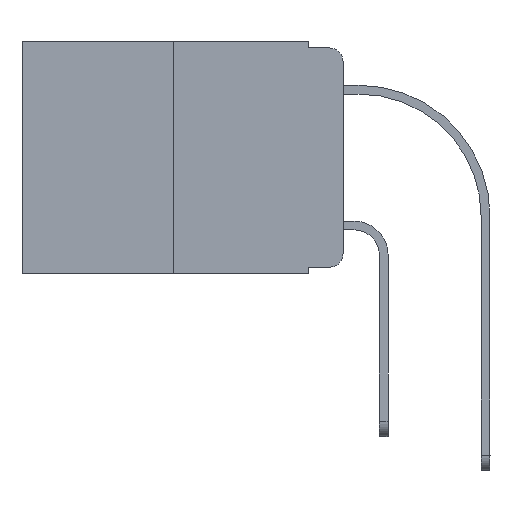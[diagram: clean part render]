
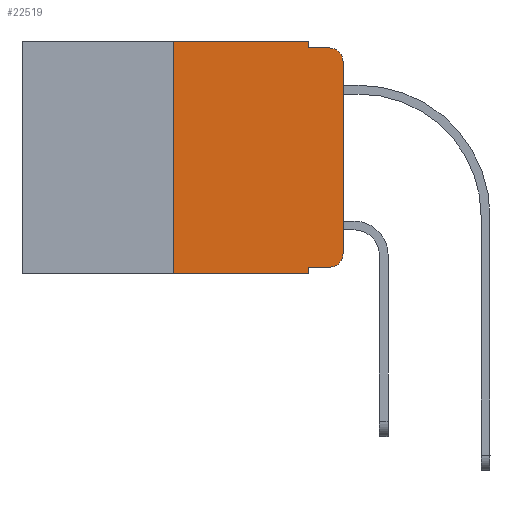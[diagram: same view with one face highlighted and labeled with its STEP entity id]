
A CAD part, left-side view. The second image highlights one B-rep face of the part: STEP entity #22519.
In plain terms, the highlighted planar face has unit normal (-1, 0, 0).
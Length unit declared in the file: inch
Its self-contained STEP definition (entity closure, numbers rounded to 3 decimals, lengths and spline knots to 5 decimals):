
#447 = DIRECTION ( 'NONE',  ( 0., -1., 0. ) ) ;
#1425 = VERTEX_POINT ( 'NONE', #23295 ) ;
#1583 = VERTEX_POINT ( 'NONE', #26199 ) ;
#2092 = CIRCLE ( 'NONE', #8124, 0.02 ) ;
#2260 = CARTESIAN_POINT ( 'NONE',  ( 0., 0.051, 0. ) ) ;
#2297 = PLANE ( 'NONE',  #5817 ) ;
#2435 = DIRECTION ( 'NONE',  ( 0., -1., 0. ) ) ;
#3812 = CIRCLE ( 'NONE', #25958, 0.02 ) ;
#4076 = FACE_OUTER_BOUND ( 'NONE', #16003, .T. ) ;
#5779 = VECTOR ( 'NONE', #447, 39.37008 ) ;
#5817 = AXIS2_PLACEMENT_3D ( 'NONE', #12988, #26584, #11105 ) ;
#6334 = DIRECTION ( 'NONE',  ( 0., 0., -1. ) ) ;
#6420 = DIRECTION ( 'NONE',  ( -1., 0., 0. ) ) ;
#6470 = ORIENTED_EDGE ( 'NONE', *, *, #17038, .T. ) ;
#6596 = DIRECTION ( 'NONE',  ( 0., -1., 0. ) ) ;
#6738 = CARTESIAN_POINT ( 'NONE',  ( 0., 0.473, -0.343 ) ) ;
#6927 = LINE ( 'NONE', #22203, #26205 ) ;
#7246 = LINE ( 'NONE', #24555, #5779 ) ;
#7475 = EDGE_CURVE ( 'NONE', #25707, #15235, #3812, .T. ) ;
#8124 = AXIS2_PLACEMENT_3D ( 'NONE', #21800, #15585, #8675 ) ;
#8242 = CARTESIAN_POINT ( 'NONE',  ( 0., 0.02, -0.333 ) ) ;
#8474 = CARTESIAN_POINT ( 'NONE',  ( 0., 0.25, 0. ) ) ;
#8675 = DIRECTION ( 'NONE',  ( 0., 0., -1. ) ) ;
#9513 = EDGE_CURVE ( 'NONE', #1425, #26608, #19741, .T. ) ;
#9763 = VERTEX_POINT ( 'NONE', #12884 ) ;
#10035 = CARTESIAN_POINT ( 'NONE',  ( 0., 0.02, -0.313 ) ) ;
#10393 = EDGE_CURVE ( 'NONE', #9763, #1425, #6927, .T. ) ;
#11105 = DIRECTION ( 'NONE',  ( 0., 0., -1. ) ) ;
#12514 = DIRECTION ( 'NONE',  ( 0., 0., 1. ) ) ;
#12521 = LINE ( 'NONE', #12937, #20308 ) ;
#12884 = CARTESIAN_POINT ( 'NONE',  ( 0., 0.25, 0. ) ) ;
#12937 = CARTESIAN_POINT ( 'NONE',  ( 0., 0.051, -0.333 ) ) ;
#12988 = CARTESIAN_POINT ( 'NONE',  ( 0., 0.473, 0. ) ) ;
#13099 = ORIENTED_EDGE ( 'NONE', *, *, #26679, .F. ) ;
#13131 = CARTESIAN_POINT ( 'NONE',  ( 0., 0.02, -0.01 ) ) ;
#13623 = VERTEX_POINT ( 'NONE', #15503 ) ;
#13699 = VECTOR ( 'NONE', #18945, 39.37008 ) ;
#14766 = VECTOR ( 'NONE', #6596, 39.37008 ) ;
#14906 = EDGE_CURVE ( 'NONE', #26608, #22482, #7246, .T. ) ;
#15203 = DIRECTION ( 'NONE',  ( 0., 0., -1. ) ) ;
#15235 = VERTEX_POINT ( 'NONE', #27881 ) ;
#15276 = ORIENTED_EDGE ( 'NONE', *, *, #7475, .T. ) ;
#15503 = CARTESIAN_POINT ( 'NONE',  ( 0., 0.051, -0.333 ) ) ;
#15552 = DIRECTION ( 'NONE',  ( 0., 0., 1. ) ) ;
#15585 = DIRECTION ( 'NONE',  ( -1., 0., 0. ) ) ;
#15869 = VECTOR ( 'NONE', #15552, 39.37008 ) ;
#16003 = EDGE_LOOP ( 'NONE', ( #27135, #27772, #20154, #28311, #24466, #23473, #20672, #13099, #6470, #15276 ) ) ;
#16338 = CARTESIAN_POINT ( 'NONE',  ( 0., 0.051, 0. ) ) ;
#17038 = EDGE_CURVE ( 'NONE', #13623, #25707, #12521, .T. ) ;
#17558 = LINE ( 'NONE', #6738, #14766 ) ;
#18360 = VECTOR ( 'NONE', #6334, 39.37008 ) ;
#18945 = DIRECTION ( 'NONE',  ( 0., 0., -1. ) ) ;
#19313 = LINE ( 'NONE', #8474, #25076 ) ;
#19741 = LINE ( 'NONE', #2260, #18360 ) ;
#20154 = ORIENTED_EDGE ( 'NONE', *, *, #14906, .F. ) ;
#20242 = EDGE_CURVE ( 'NONE', #1583, #9763, #19313, .T. ) ;
#20308 = VECTOR ( 'NONE', #21754, 39.37008 ) ;
#20672 = ORIENTED_EDGE ( 'NONE', *, *, #21698, .T. ) ;
#20710 = VERTEX_POINT ( 'NONE', #28192 ) ;
#21633 = CARTESIAN_POINT ( 'NONE',  ( 0., 0., 0. ) ) ;
#21698 = EDGE_CURVE ( 'NONE', #1583, #23809, #17558, .T. ) ;
#21704 = CARTESIAN_POINT ( 'NONE',  ( 0., 0.051, -0.343 ) ) ;
#21754 = DIRECTION ( 'NONE',  ( 0., -1., 0. ) ) ;
#21800 = CARTESIAN_POINT ( 'NONE',  ( 0., 0.02, -0.03 ) ) ;
#21897 = LINE ( 'NONE', #21633, #15869 ) ;
#22203 = CARTESIAN_POINT ( 'NONE',  ( 0., 0.473, 0. ) ) ;
#22482 = VERTEX_POINT ( 'NONE', #13131 ) ;
#22519 = ADVANCED_FACE ( 'NONE', ( #4076 ), #2297, .F. ) ;
#22526 = EDGE_CURVE ( 'NONE', #20710, #22482, #2092, .T. ) ;
#22957 = EDGE_CURVE ( 'NONE', #15235, #20710, #21897, .T. ) ;
#23295 = CARTESIAN_POINT ( 'NONE',  ( 0., 0.051, 0. ) ) ;
#23473 = ORIENTED_EDGE ( 'NONE', *, *, #20242, .F. ) ;
#23809 = VERTEX_POINT ( 'NONE', #21704 ) ;
#24292 = LINE ( 'NONE', #16338, #13699 ) ;
#24466 = ORIENTED_EDGE ( 'NONE', *, *, #10393, .F. ) ;
#24555 = CARTESIAN_POINT ( 'NONE',  ( 0., 0.051, -0.01 ) ) ;
#24879 = CARTESIAN_POINT ( 'NONE',  ( 0., 0.051, -0.01 ) ) ;
#25076 = VECTOR ( 'NONE', #12514, 39.37008 ) ;
#25707 = VERTEX_POINT ( 'NONE', #8242 ) ;
#25958 = AXIS2_PLACEMENT_3D ( 'NONE', #10035, #6420, #15203 ) ;
#26199 = CARTESIAN_POINT ( 'NONE',  ( 0., 0.25, -0.343 ) ) ;
#26205 = VECTOR ( 'NONE', #2435, 39.37008 ) ;
#26584 = DIRECTION ( 'NONE',  ( 1., 0., 0. ) ) ;
#26608 = VERTEX_POINT ( 'NONE', #24879 ) ;
#26679 = EDGE_CURVE ( 'NONE', #13623, #23809, #24292, .T. ) ;
#27135 = ORIENTED_EDGE ( 'NONE', *, *, #22957, .T. ) ;
#27772 = ORIENTED_EDGE ( 'NONE', *, *, #22526, .T. ) ;
#27881 = CARTESIAN_POINT ( 'NONE',  ( 0., 0., -0.313 ) ) ;
#28192 = CARTESIAN_POINT ( 'NONE',  ( 0., 0., -0.03 ) ) ;
#28311 = ORIENTED_EDGE ( 'NONE', *, *, #9513, .F. ) ;
